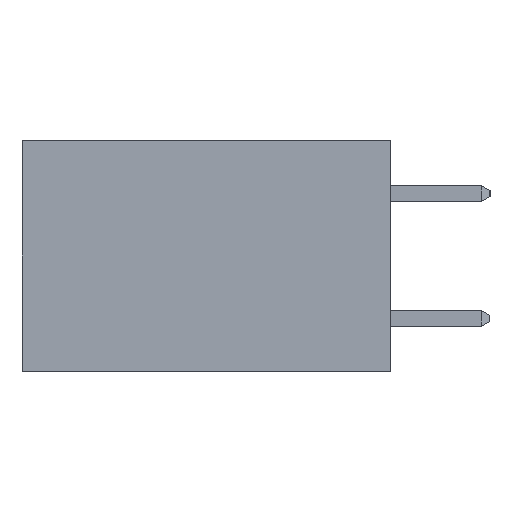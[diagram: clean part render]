
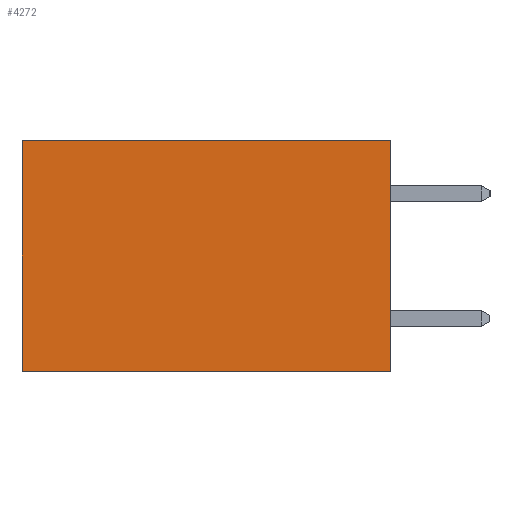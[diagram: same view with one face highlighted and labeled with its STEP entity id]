
A CAD part, left-side view. The second image highlights one B-rep face of the part: STEP entity #4272.
In plain terms, the highlighted planar face has unit normal (-1, 0, 0).
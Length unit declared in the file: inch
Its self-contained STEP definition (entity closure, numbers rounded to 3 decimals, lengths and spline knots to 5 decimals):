
#122 = CARTESIAN_POINT ( 'NONE',  ( 0.277, 0., -0.37 ) ) ;
#449 = DIRECTION ( 'NONE',  ( 0., 1., 0. ) ) ;
#450 = ORIENTED_EDGE ( 'NONE', *, *, #554, .T. ) ;
#554 = EDGE_CURVE ( 'NONE', #9026, #8919, #5042, .T. ) ;
#569 = LINE ( 'NONE', #122, #3522 ) ;
#1016 = CARTESIAN_POINT ( 'NONE',  ( 0.277, 0.59, -0.37 ) ) ;
#1029 = CARTESIAN_POINT ( 'NONE',  ( 0.277, 0.59, -0.37 ) ) ;
#1387 = CARTESIAN_POINT ( 'NONE',  ( 0.277, 0., 0. ) ) ;
#1390 = CARTESIAN_POINT ( 'NONE',  ( 0.277, 0., 0. ) ) ;
#1659 = LINE ( 'NONE', #1016, #11854 ) ;
#2776 = ORIENTED_EDGE ( 'NONE', *, *, #10193, .F. ) ;
#2973 = DIRECTION ( 'NONE',  ( 0., 0., -1. ) ) ;
#3522 = VECTOR ( 'NONE', #12691, 39.37008 ) ;
#4250 = CARTESIAN_POINT ( 'NONE',  ( 0.277, 0.59, 0. ) ) ;
#4272 = ADVANCED_FACE ( 'NONE', ( #11734 ), #9646, .F. ) ;
#5042 = LINE ( 'NONE', #1390, #9978 ) ;
#5084 = EDGE_CURVE ( 'NONE', #9026, #11658, #569, .T. ) ;
#6260 = CARTESIAN_POINT ( 'NONE',  ( 0.277, 0., -0.37 ) ) ;
#6470 = EDGE_LOOP ( 'NONE', ( #10061, #2776, #8056, #450 ) ) ;
#7415 = CARTESIAN_POINT ( 'NONE',  ( 0.277, 0., -0.37 ) ) ;
#7760 = AXIS2_PLACEMENT_3D ( 'NONE', #9048, #9018, #8959 ) ;
#8004 = VERTEX_POINT ( 'NONE', #1029 ) ;
#8056 = ORIENTED_EDGE ( 'NONE', *, *, #5084, .F. ) ;
#8487 = VECTOR ( 'NONE', #449, 39.37008 ) ;
#8542 = DIRECTION ( 'NONE',  ( 0., 1., 0. ) ) ;
#8919 = VERTEX_POINT ( 'NONE', #4250 ) ;
#8959 = DIRECTION ( 'NONE',  ( 0., 0., -1. ) ) ;
#9018 = DIRECTION ( 'NONE',  ( 1., 0., 0. ) ) ;
#9026 = VERTEX_POINT ( 'NONE', #1387 ) ;
#9048 = CARTESIAN_POINT ( 'NONE',  ( 0.277, 0., -0.37 ) ) ;
#9646 = PLANE ( 'NONE',  #7760 ) ;
#9978 = VECTOR ( 'NONE', #8542, 39.37008 ) ;
#10061 = ORIENTED_EDGE ( 'NONE', *, *, #12645, .T. ) ;
#10193 = EDGE_CURVE ( 'NONE', #11658, #8004, #11089, .T. ) ;
#11089 = LINE ( 'NONE', #7415, #8487 ) ;
#11658 = VERTEX_POINT ( 'NONE', #6260 ) ;
#11734 = FACE_OUTER_BOUND ( 'NONE', #6470, .T. ) ;
#11854 = VECTOR ( 'NONE', #2973, 39.37008 ) ;
#12645 = EDGE_CURVE ( 'NONE', #8919, #8004, #1659, .T. ) ;
#12691 = DIRECTION ( 'NONE',  ( 0., 0., -1. ) ) ;
